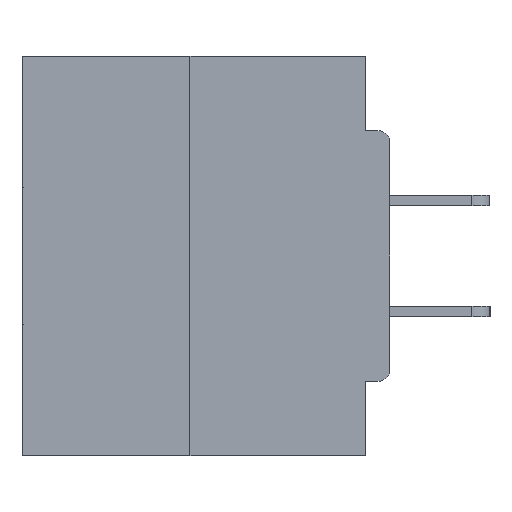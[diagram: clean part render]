
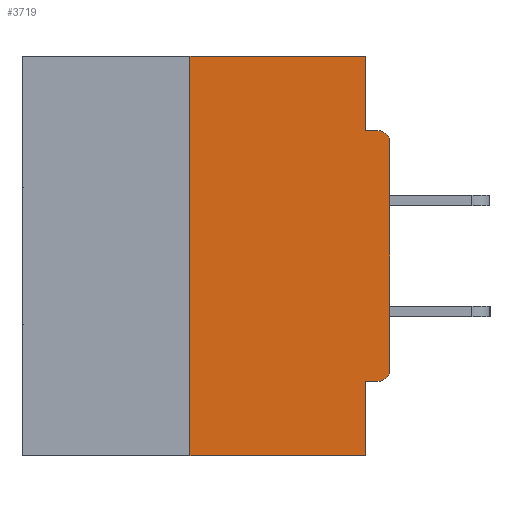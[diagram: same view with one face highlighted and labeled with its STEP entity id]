
A CAD part, left-side view. The second image highlights one B-rep face of the part: STEP entity #3719.
In plain terms, the highlighted planar face has unit normal (-1, 0, 0).
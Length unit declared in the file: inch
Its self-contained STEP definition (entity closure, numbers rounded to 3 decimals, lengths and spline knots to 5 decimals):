
#457 = DIRECTION ( 'NONE',  ( -1., 0., 0. ) ) ;
#1361 = CARTESIAN_POINT ( 'NONE',  ( 0., 0.031, -0.0935 ) ) ;
#1604 = VECTOR ( 'NONE', #25961, 39.37008 ) ;
#1657 = LINE ( 'NONE', #21884, #35346 ) ;
#1828 = DIRECTION ( 'NONE',  ( 0., 0., -1. ) ) ;
#1869 = CARTESIAN_POINT ( 'NONE',  ( 0., 0., -0.3915 ) ) ;
#2200 = CARTESIAN_POINT ( 'NONE',  ( 0., 0.015, -0.1085 ) ) ;
#2878 = EDGE_CURVE ( 'NONE', #33176, #8810, #26851, .T. ) ;
#3469 = VERTEX_POINT ( 'NONE', #18107 ) ;
#3637 = EDGE_CURVE ( 'NONE', #29262, #35275, #25832, .T. ) ;
#3719 = ADVANCED_FACE ( 'NONE', ( #22565 ), #22358, .F. ) ;
#3977 = EDGE_CURVE ( 'NONE', #34864, #8042, #27539, .T. ) ;
#4574 = EDGE_CURVE ( 'NONE', #34864, #31777, #1657, .T. ) ;
#4675 = EDGE_LOOP ( 'NONE', ( #27734, #17090, #32396, #20919, #35009, #28988, #18066, #10886, #12349, #12194 ) ) ;
#4957 = LINE ( 'NONE', #22708, #25606 ) ;
#5623 = CARTESIAN_POINT ( 'NONE',  ( 0., 0.25, 0. ) ) ;
#5855 = DIRECTION ( 'NONE',  ( 0., 0., -1. ) ) ;
#6171 = EDGE_CURVE ( 'NONE', #32109, #8042, #19705, .T. ) ;
#7533 = DIRECTION ( 'NONE',  ( 0., 0., -1. ) ) ;
#7540 = CARTESIAN_POINT ( 'NONE',  ( 0., 0.031, -0.4065 ) ) ;
#7879 = CARTESIAN_POINT ( 'NONE',  ( 0., 0.031, 0. ) ) ;
#8042 = VERTEX_POINT ( 'NONE', #25782 ) ;
#8583 = EDGE_CURVE ( 'NONE', #33176, #32109, #18146, .T. ) ;
#8810 = VERTEX_POINT ( 'NONE', #1869 ) ;
#9975 = VECTOR ( 'NONE', #10167, 39.37008 ) ;
#10167 = DIRECTION ( 'NONE',  ( 0., -1., 0. ) ) ;
#10793 = VERTEX_POINT ( 'NONE', #18366 ) ;
#10856 = AXIS2_PLACEMENT_3D ( 'NONE', #29197, #457, #5855 ) ;
#10886 = ORIENTED_EDGE ( 'NONE', *, *, #21251, .T. ) ;
#11301 = VECTOR ( 'NONE', #13320, 39.37008 ) ;
#12142 = DIRECTION ( 'NONE',  ( 0., -1., 0. ) ) ;
#12194 = ORIENTED_EDGE ( 'NONE', *, *, #15500, .F. ) ;
#12349 = ORIENTED_EDGE ( 'NONE', *, *, #3637, .F. ) ;
#13320 = DIRECTION ( 'NONE',  ( 0., -1., 0. ) ) ;
#13880 = DIRECTION ( 'NONE',  ( 1., 0., 0. ) ) ;
#13938 = CARTESIAN_POINT ( 'NONE',  ( 0., 0.031, -0.5 ) ) ;
#14363 = VECTOR ( 'NONE', #12142, 39.37008 ) ;
#14510 = DIRECTION ( 'NONE',  ( 0., 0., -1. ) ) ;
#15500 = EDGE_CURVE ( 'NONE', #3469, #29262, #19976, .T. ) ;
#15596 = EDGE_CURVE ( 'NONE', #8810, #10793, #4957, .T. ) ;
#16309 = CARTESIAN_POINT ( 'NONE',  ( 0., 0.46, 0. ) ) ;
#16897 = DIRECTION ( 'NONE',  ( 0., 0., 1. ) ) ;
#17090 = ORIENTED_EDGE ( 'NONE', *, *, #4574, .F. ) ;
#18066 = ORIENTED_EDGE ( 'NONE', *, *, #15596, .T. ) ;
#18107 = CARTESIAN_POINT ( 'NONE',  ( 0., 0.031, 0. ) ) ;
#18146 = LINE ( 'NONE', #29739, #20348 ) ;
#18366 = CARTESIAN_POINT ( 'NONE',  ( 0., 0., -0.1085 ) ) ;
#19705 = LINE ( 'NONE', #13938, #34812 ) ;
#19976 = LINE ( 'NONE', #7879, #1604 ) ;
#20348 = VECTOR ( 'NONE', #29188, 39.37008 ) ;
#20919 = ORIENTED_EDGE ( 'NONE', *, *, #6171, .F. ) ;
#21251 = EDGE_CURVE ( 'NONE', #10793, #35275, #34142, .T. ) ;
#21884 = CARTESIAN_POINT ( 'NONE',  ( 0., 0.25, 0. ) ) ;
#22358 = PLANE ( 'NONE',  #29113 ) ;
#22565 = FACE_OUTER_BOUND ( 'NONE', #4675, .T. ) ;
#22708 = CARTESIAN_POINT ( 'NONE',  ( 0., 0., 0. ) ) ;
#23070 = AXIS2_PLACEMENT_3D ( 'NONE', #2200, #31313, #1828 ) ;
#24448 = CARTESIAN_POINT ( 'NONE',  ( 0., 0.015, -0.0935 ) ) ;
#24785 = LINE ( 'NONE', #16309, #9975 ) ;
#25606 = VECTOR ( 'NONE', #16897, 39.37008 ) ;
#25782 = CARTESIAN_POINT ( 'NONE',  ( 0., 0.031, -0.5 ) ) ;
#25832 = LINE ( 'NONE', #37599, #11301 ) ;
#25961 = DIRECTION ( 'NONE',  ( 0., 0., -1. ) ) ;
#26851 = CIRCLE ( 'NONE', #10856, 0.015 ) ;
#27539 = LINE ( 'NONE', #30049, #14363 ) ;
#27734 = ORIENTED_EDGE ( 'NONE', *, *, #32909, .F. ) ;
#28988 = ORIENTED_EDGE ( 'NONE', *, *, #2878, .T. ) ;
#29113 = AXIS2_PLACEMENT_3D ( 'NONE', #34317, #13880, #7533 ) ;
#29188 = DIRECTION ( 'NONE',  ( 0., 1., 0. ) ) ;
#29197 = CARTESIAN_POINT ( 'NONE',  ( 0., 0.015, -0.3915 ) ) ;
#29262 = VERTEX_POINT ( 'NONE', #1361 ) ;
#29413 = CARTESIAN_POINT ( 'NONE',  ( 0., 0.015, -0.4065 ) ) ;
#29739 = CARTESIAN_POINT ( 'NONE',  ( 0., 0., -0.4065 ) ) ;
#30049 = CARTESIAN_POINT ( 'NONE',  ( 0., 0.46, -0.5 ) ) ;
#30575 = DIRECTION ( 'NONE',  ( 0., 0., 1. ) ) ;
#31313 = DIRECTION ( 'NONE',  ( -1., 0., 0. ) ) ;
#31777 = VERTEX_POINT ( 'NONE', #5623 ) ;
#32109 = VERTEX_POINT ( 'NONE', #7540 ) ;
#32396 = ORIENTED_EDGE ( 'NONE', *, *, #3977, .T. ) ;
#32441 = CARTESIAN_POINT ( 'NONE',  ( 0., 0.25, -0.5 ) ) ;
#32909 = EDGE_CURVE ( 'NONE', #31777, #3469, #24785, .T. ) ;
#33176 = VERTEX_POINT ( 'NONE', #29413 ) ;
#34142 = CIRCLE ( 'NONE', #23070, 0.015 ) ;
#34317 = CARTESIAN_POINT ( 'NONE',  ( 0., 0.46, 0. ) ) ;
#34812 = VECTOR ( 'NONE', #14510, 39.37008 ) ;
#34864 = VERTEX_POINT ( 'NONE', #32441 ) ;
#35009 = ORIENTED_EDGE ( 'NONE', *, *, #8583, .F. ) ;
#35275 = VERTEX_POINT ( 'NONE', #24448 ) ;
#35346 = VECTOR ( 'NONE', #30575, 39.37008 ) ;
#37599 = CARTESIAN_POINT ( 'NONE',  ( 0., 0., -0.0935 ) ) ;
